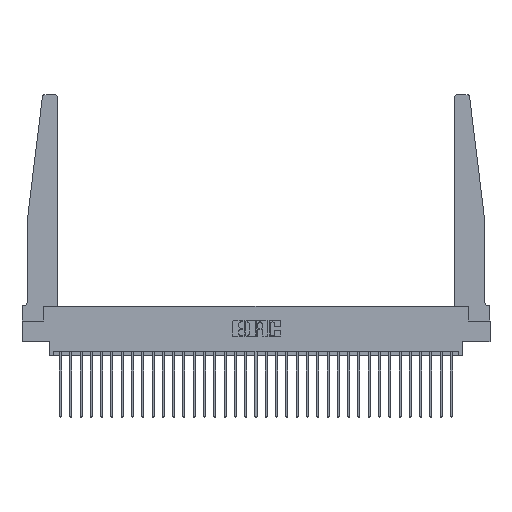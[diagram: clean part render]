
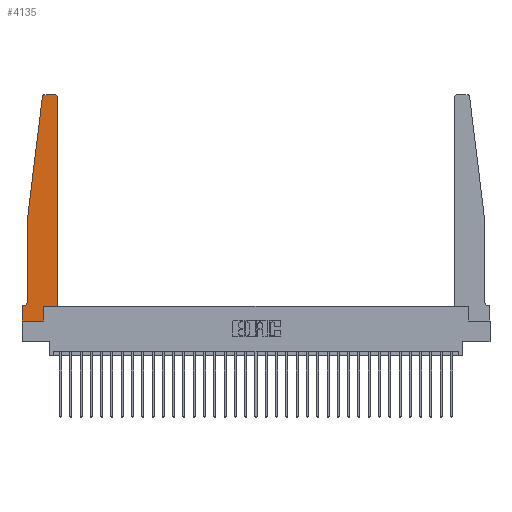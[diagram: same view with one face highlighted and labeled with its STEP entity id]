
A CAD part, top view. The second image highlights one B-rep face of the part: STEP entity #4135.
In plain terms, the highlighted planar face has unit normal (0, 0, 1).
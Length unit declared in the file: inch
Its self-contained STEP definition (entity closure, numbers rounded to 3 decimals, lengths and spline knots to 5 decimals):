
#395 = LINE ( 'NONE', #11942, #23582 ) ;
#462 = ORIENTED_EDGE ( 'NONE', *, *, #24277, .T. ) ;
#1553 = DIRECTION ( 'NONE',  ( 1., 0., 0. ) ) ;
#1667 = CARTESIAN_POINT ( 'NONE',  ( 0.425, 0.18, 0.37 ) ) ;
#1837 = DIRECTION ( 'NONE',  ( -0.122, -0.992, 0. ) ) ;
#2011 = PLANE ( 'NONE',  #12841 ) ;
#2014 = CARTESIAN_POINT ( 'NONE',  ( 0., 0.1875, 0.37 ) ) ;
#2062 = EDGE_CURVE ( 'NONE', #10839, #25734, #21006, .T. ) ;
#2203 = VECTOR ( 'NONE', #16751, 39.37008 ) ;
#2614 = VECTOR ( 'NONE', #13371, 39.37008 ) ;
#2648 = CARTESIAN_POINT ( 'NONE',  ( 0.065, 0.2375, 0.37 ) ) ;
#3140 = VERTEX_POINT ( 'NONE', #24187 ) ;
#3644 = VECTOR ( 'NONE', #12856, 39.37008 ) ;
#3926 = FACE_OUTER_BOUND ( 'NONE', #20903, .T. ) ;
#3941 = DIRECTION ( 'NONE',  ( -1., 0., 0. ) ) ;
#4135 = ADVANCED_FACE ( 'NONE', ( #3926 ), #2011, .T. ) ;
#5737 = LINE ( 'NONE', #24577, #20291 ) ;
#6089 = DIRECTION ( 'NONE',  ( 0., -1., 0. ) ) ;
#6390 = CARTESIAN_POINT ( 'NONE',  ( 0.395, 2.75, 0.37 ) ) ;
#6593 = ORIENTED_EDGE ( 'NONE', *, *, #18043, .T. ) ;
#7674 = EDGE_CURVE ( 'NONE', #22465, #29660, #395, .T. ) ;
#8166 = CARTESIAN_POINT ( 'NONE',  ( 0.2605, 0.18, 0.37 ) ) ;
#8826 = DIRECTION ( 'NONE',  ( 0., 0., 1. ) ) ;
#8852 = VECTOR ( 'NONE', #14018, 39.37008 ) ;
#9399 = ORIENTED_EDGE ( 'NONE', *, *, #14525, .T. ) ;
#9891 = CARTESIAN_POINT ( 'NONE',  ( 0.425, 0.18, 0.37 ) ) ;
#9906 = ORIENTED_EDGE ( 'NONE', *, *, #2062, .T. ) ;
#10427 = VECTOR ( 'NONE', #3941, 39.37008 ) ;
#10709 = CARTESIAN_POINT ( 'NONE',  ( 0.27653, 2.75, 0.37 ) ) ;
#10773 = ORIENTED_EDGE ( 'NONE', *, *, #20881, .T. ) ;
#10839 = VERTEX_POINT ( 'NONE', #23581 ) ;
#10960 = VERTEX_POINT ( 'NONE', #24211 ) ;
#11062 = DIRECTION ( 'NONE',  ( 0., 0., -1. ) ) ;
#11653 = DIRECTION ( 'NONE',  ( 1., 0., 0. ) ) ;
#11672 = LINE ( 'NONE', #13735, #2203 ) ;
#11942 = CARTESIAN_POINT ( 'NONE',  ( 0.425, 0.18, 0.37 ) ) ;
#12841 = AXIS2_PLACEMENT_3D ( 'NONE', #30474, #8826, #11653 ) ;
#12843 = CIRCLE ( 'NONE', #16910, 0.03 ) ;
#12856 = DIRECTION ( 'NONE',  ( 0., 1., 0. ) ) ;
#13048 = CARTESIAN_POINT ( 'NONE',  ( 0., 0., 0.37 ) ) ;
#13371 = DIRECTION ( 'NONE',  ( 1., 0., 0. ) ) ;
#13735 = CARTESIAN_POINT ( 'NONE',  ( 0.065, 1.25, 0.37 ) ) ;
#14018 = DIRECTION ( 'NONE',  ( 0., 1., 0. ) ) ;
#14326 = EDGE_CURVE ( 'NONE', #3140, #23665, #20959, .T. ) ;
#14416 = VECTOR ( 'NONE', #1837, 39.37008 ) ;
#14525 = EDGE_CURVE ( 'NONE', #23665, #22465, #19998, .T. ) ;
#14580 = EDGE_CURVE ( 'NONE', #18970, #17243, #5737, .T. ) ;
#15137 = ORIENTED_EDGE ( 'NONE', *, *, #7674, .T. ) ;
#15259 = CARTESIAN_POINT ( 'NONE',  ( 0.065, 1.25, 0.37 ) ) ;
#15747 = LINE ( 'NONE', #13048, #29703 ) ;
#15963 = CARTESIAN_POINT ( 'NONE',  ( 0.27653, 2.72, 0.37 ) ) ;
#16414 = CARTESIAN_POINT ( 'NONE',  ( 0.065, 0.1875, 0.37 ) ) ;
#16751 = DIRECTION ( 'NONE',  ( 0., -1., 0. ) ) ;
#16902 = EDGE_CURVE ( 'NONE', #29622, #31002, #11672, .T. ) ;
#16910 = AXIS2_PLACEMENT_3D ( 'NONE', #15963, #18339, #1553 ) ;
#17243 = VERTEX_POINT ( 'NONE', #10709 ) ;
#18043 = EDGE_CURVE ( 'NONE', #17243, #30917, #12843, .T. ) ;
#18339 = DIRECTION ( 'NONE',  ( 0., 0., 1. ) ) ;
#18633 = EDGE_CURVE ( 'NONE', #29660, #10960, #23352, .T. ) ;
#18662 = ORIENTED_EDGE ( 'NONE', *, *, #19347, .T. ) ;
#18970 = VERTEX_POINT ( 'NONE', #6390 ) ;
#19054 = ORIENTED_EDGE ( 'NONE', *, *, #14326, .T. ) ;
#19319 = CARTESIAN_POINT ( 'NONE',  ( 0.395, 2.72, 0.37 ) ) ;
#19347 = EDGE_CURVE ( 'NONE', #31002, #10839, #23961, .T. ) ;
#19686 = CARTESIAN_POINT ( 'NONE',  ( 0.2605, 0.18, 0.37 ) ) ;
#19998 = LINE ( 'NONE', #19686, #3644 ) ;
#20291 = VECTOR ( 'NONE', #29320, 39.37008 ) ;
#20388 = AXIS2_PLACEMENT_3D ( 'NONE', #19319, #28958, #24372 ) ;
#20395 = CARTESIAN_POINT ( 'NONE',  ( 0.015, 0.2375, 0.37 ) ) ;
#20881 = EDGE_CURVE ( 'NONE', #30917, #29622, #21751, .T. ) ;
#20903 = EDGE_LOOP ( 'NONE', ( #21119, #6593, #10773, #22135, #18662, #9906, #462, #19054, #9399, #15137, #24298, #25198 ) ) ;
#20959 = LINE ( 'NONE', #28389, #2614 ) ;
#21006 = LINE ( 'NONE', #16414, #10427 ) ;
#21119 = ORIENTED_EDGE ( 'NONE', *, *, #14580, .T. ) ;
#21434 = AXIS2_PLACEMENT_3D ( 'NONE', #20395, #11062, #30044 ) ;
#21751 = LINE ( 'NONE', #26338, #14416 ) ;
#22135 = ORIENTED_EDGE ( 'NONE', *, *, #16902, .T. ) ;
#22465 = VERTEX_POINT ( 'NONE', #8166 ) ;
#23352 = LINE ( 'NONE', #1667, #8852 ) ;
#23581 = CARTESIAN_POINT ( 'NONE',  ( 0.015, 0.1875, 0.37 ) ) ;
#23582 = VECTOR ( 'NONE', #29480, 39.37008 ) ;
#23665 = VERTEX_POINT ( 'NONE', #23860 ) ;
#23860 = CARTESIAN_POINT ( 'NONE',  ( 0.2605, 0., 0.37 ) ) ;
#23924 = CIRCLE ( 'NONE', #20388, 0.03 ) ;
#23961 = CIRCLE ( 'NONE', #21434, 0.05 ) ;
#24187 = CARTESIAN_POINT ( 'NONE',  ( 0., 0., 0.37 ) ) ;
#24211 = CARTESIAN_POINT ( 'NONE',  ( 0.425, 2.72, 0.37 ) ) ;
#24277 = EDGE_CURVE ( 'NONE', #25734, #3140, #15747, .T. ) ;
#24298 = ORIENTED_EDGE ( 'NONE', *, *, #18633, .T. ) ;
#24372 = DIRECTION ( 'NONE',  ( 1., 0., 0. ) ) ;
#24577 = CARTESIAN_POINT ( 'NONE',  ( 0.25, 2.75, 0.37 ) ) ;
#25198 = ORIENTED_EDGE ( 'NONE', *, *, #26291, .T. ) ;
#25734 = VERTEX_POINT ( 'NONE', #2014 ) ;
#26291 = EDGE_CURVE ( 'NONE', #10960, #18970, #23924, .T. ) ;
#26338 = CARTESIAN_POINT ( 'NONE',  ( 0.065, 1.25, 0.37 ) ) ;
#26522 = CARTESIAN_POINT ( 'NONE',  ( 0.24675, 2.72367, 0.37 ) ) ;
#28389 = CARTESIAN_POINT ( 'NONE',  ( 0., 0., 0.37 ) ) ;
#28958 = DIRECTION ( 'NONE',  ( 0., 0., 1. ) ) ;
#29320 = DIRECTION ( 'NONE',  ( -1., 0., 0. ) ) ;
#29480 = DIRECTION ( 'NONE',  ( 1., 0., 0. ) ) ;
#29622 = VERTEX_POINT ( 'NONE', #15259 ) ;
#29660 = VERTEX_POINT ( 'NONE', #9891 ) ;
#29703 = VECTOR ( 'NONE', #6089, 39.37008 ) ;
#30044 = DIRECTION ( 'NONE',  ( -1., 0., 0. ) ) ;
#30474 = CARTESIAN_POINT ( 'NONE',  ( 0., 0.1875, 0.37 ) ) ;
#30917 = VERTEX_POINT ( 'NONE', #26522 ) ;
#31002 = VERTEX_POINT ( 'NONE', #2648 ) ;
